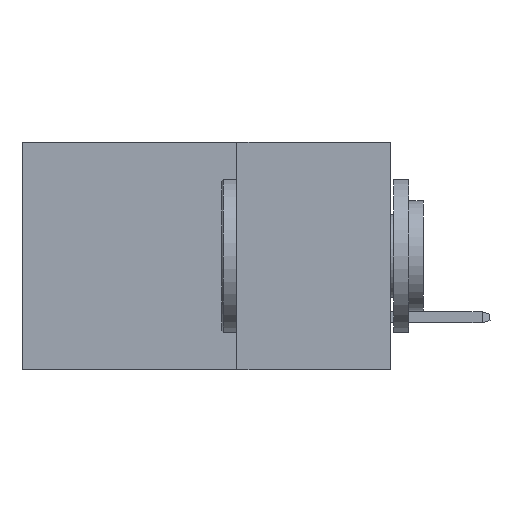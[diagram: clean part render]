
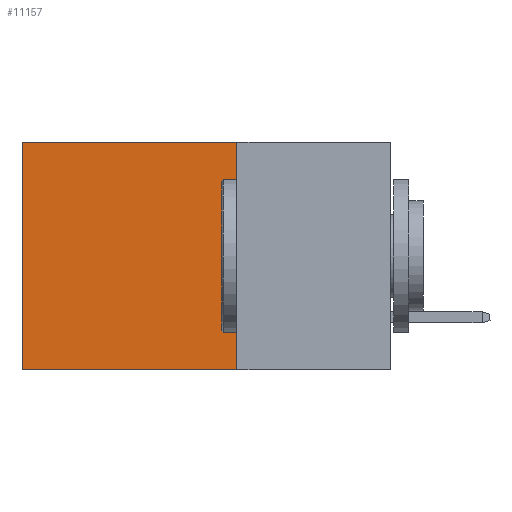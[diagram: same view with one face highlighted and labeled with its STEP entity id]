
A CAD part, left-side view. The second image highlights one B-rep face of the part: STEP entity #11157.
In plain terms, the highlighted planar face has unit normal (-1, 0, 0).
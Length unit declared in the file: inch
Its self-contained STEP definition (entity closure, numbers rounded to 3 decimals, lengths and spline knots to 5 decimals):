
#566 = EDGE_CURVE ( 'NONE', #7464, #17622, #4731, .T. ) ;
#1202 = VERTEX_POINT ( 'NONE', #6963 ) ;
#2769 = CARTESIAN_POINT ( 'NONE',  ( 0.2875, 0.25, -0.37 ) ) ;
#3144 = DIRECTION ( 'NONE',  ( 0., 0., -1. ) ) ;
#3273 = VECTOR ( 'NONE', #4442, 39.37008 ) ;
#3357 = DIRECTION ( 'NONE',  ( 1., 0., 0. ) ) ;
#4442 = DIRECTION ( 'NONE',  ( 0., 1., 0. ) ) ;
#4731 = LINE ( 'NONE', #10273, #8014 ) ;
#6963 = CARTESIAN_POINT ( 'NONE',  ( 0.2875, 0.6, -0.37 ) ) ;
#7248 = ORIENTED_EDGE ( 'NONE', *, *, #566, .F. ) ;
#7362 = EDGE_CURVE ( 'NONE', #8122, #1202, #10697, .T. ) ;
#7464 = VERTEX_POINT ( 'NONE', #18005 ) ;
#8014 = VECTOR ( 'NONE', #3144, 39.37008 ) ;
#8122 = VERTEX_POINT ( 'NONE', #15326 ) ;
#8162 = EDGE_CURVE ( 'NONE', #7464, #8122, #10765, .T. ) ;
#8415 = DIRECTION ( 'NONE',  ( 0., 0., -1. ) ) ;
#8625 = CARTESIAN_POINT ( 'NONE',  ( 0.2875, 0.25, 0. ) ) ;
#8908 = CARTESIAN_POINT ( 'NONE',  ( 0.2875, 0.25, -0.37 ) ) ;
#8992 = PLANE ( 'NONE',  #14456 ) ;
#10273 = CARTESIAN_POINT ( 'NONE',  ( 0.2875, 0.25, 0. ) ) ;
#10642 = FACE_OUTER_BOUND ( 'NONE', #16111, .T. ) ;
#10697 = LINE ( 'NONE', #15185, #17384 ) ;
#10765 = LINE ( 'NONE', #8625, #3273 ) ;
#11157 = ADVANCED_FACE ( 'NONE', ( #10642 ), #8992, .F. ) ;
#12270 = EDGE_CURVE ( 'NONE', #17622, #1202, #14449, .T. ) ;
#13039 = ORIENTED_EDGE ( 'NONE', *, *, #7362, .T. ) ;
#13089 = CARTESIAN_POINT ( 'NONE',  ( 0.2875, 0.25, 0. ) ) ;
#13148 = DIRECTION ( 'NONE',  ( 0., 0., -1. ) ) ;
#13636 = VECTOR ( 'NONE', #14013, 39.37008 ) ;
#14013 = DIRECTION ( 'NONE',  ( 0., 1., 0. ) ) ;
#14449 = LINE ( 'NONE', #2769, #13636 ) ;
#14456 = AXIS2_PLACEMENT_3D ( 'NONE', #13089, #3357, #13148 ) ;
#14953 = ORIENTED_EDGE ( 'NONE', *, *, #8162, .T. ) ;
#15185 = CARTESIAN_POINT ( 'NONE',  ( 0.2875, 0.6, 0. ) ) ;
#15326 = CARTESIAN_POINT ( 'NONE',  ( 0.2875, 0.6, 0. ) ) ;
#16111 = EDGE_LOOP ( 'NONE', ( #13039, #17348, #7248, #14953 ) ) ;
#17348 = ORIENTED_EDGE ( 'NONE', *, *, #12270, .F. ) ;
#17384 = VECTOR ( 'NONE', #8415, 39.37008 ) ;
#17622 = VERTEX_POINT ( 'NONE', #8908 ) ;
#18005 = CARTESIAN_POINT ( 'NONE',  ( 0.2875, 0.25, 0. ) ) ;
